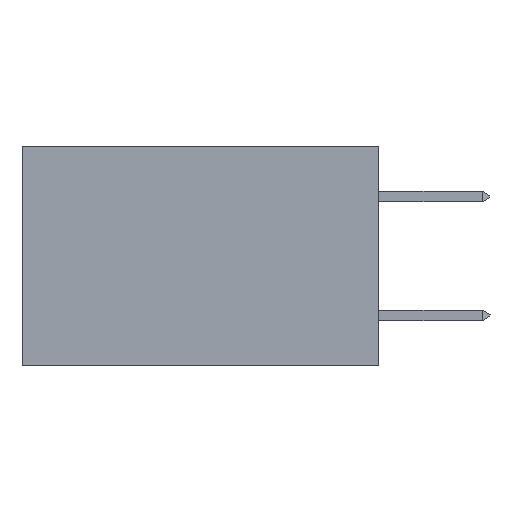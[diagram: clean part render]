
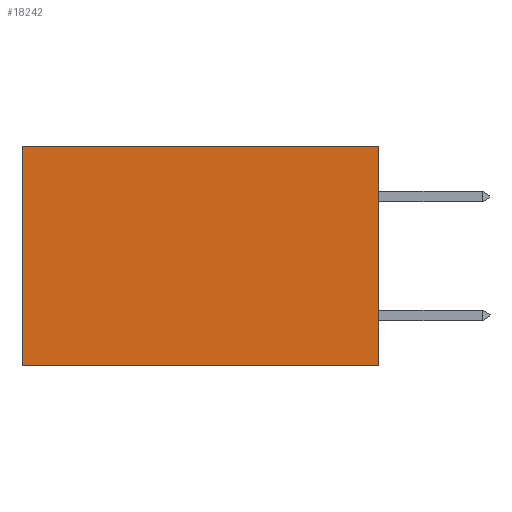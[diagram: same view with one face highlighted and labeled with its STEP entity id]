
A CAD part, left-side view. The second image highlights one B-rep face of the part: STEP entity #18242.
In plain terms, the highlighted planar face has unit normal (-1, 0, 0).
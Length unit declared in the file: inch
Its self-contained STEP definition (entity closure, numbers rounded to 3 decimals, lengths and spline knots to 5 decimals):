
#259 = VERTEX_POINT ( 'NONE', #22582 ) ;
#713 = CARTESIAN_POINT ( 'NONE',  ( 0.298, 0., 0. ) ) ;
#2427 = DIRECTION ( 'NONE',  ( 0., 1., 0. ) ) ;
#2491 = ORIENTED_EDGE ( 'NONE', *, *, #16410, .F. ) ;
#2570 = LINE ( 'NONE', #713, #17708 ) ;
#2868 = EDGE_CURVE ( 'NONE', #259, #24643, #7795, .T. ) ;
#3709 = VECTOR ( 'NONE', #2427, 39.37008 ) ;
#3842 = CARTESIAN_POINT ( 'NONE',  ( 0.298, 0., 0. ) ) ;
#5286 = FACE_OUTER_BOUND ( 'NONE', #17323, .T. ) ;
#5884 = VERTEX_POINT ( 'NONE', #3842 ) ;
#6358 = CARTESIAN_POINT ( 'NONE',  ( 0.298, 0., -0.37 ) ) ;
#7116 = AXIS2_PLACEMENT_3D ( 'NONE', #25518, #19274, #10791 ) ;
#7795 = LINE ( 'NONE', #15834, #25269 ) ;
#8068 = CARTESIAN_POINT ( 'NONE',  ( 0.298, 0., 0. ) ) ;
#10046 = VERTEX_POINT ( 'NONE', #6358 ) ;
#10791 = DIRECTION ( 'NONE',  ( 0., 0., -1. ) ) ;
#10875 = CARTESIAN_POINT ( 'NONE',  ( 0.298, 0., -0.37 ) ) ;
#12385 = ORIENTED_EDGE ( 'NONE', *, *, #26839, .F. ) ;
#12561 = EDGE_CURVE ( 'NONE', #5884, #259, #2570, .T. ) ;
#14695 = ORIENTED_EDGE ( 'NONE', *, *, #2868, .T. ) ;
#14833 = PLANE ( 'NONE',  #7116 ) ;
#15834 = CARTESIAN_POINT ( 'NONE',  ( 0.298, 0.6, 0. ) ) ;
#16410 = EDGE_CURVE ( 'NONE', #10046, #24643, #21798, .T. ) ;
#16470 = DIRECTION ( 'NONE',  ( 0., 0., -1. ) ) ;
#17323 = EDGE_LOOP ( 'NONE', ( #14695, #2491, #12385, #21413 ) ) ;
#17708 = VECTOR ( 'NONE', #19185, 39.37008 ) ;
#18242 = ADVANCED_FACE ( 'NONE', ( #5286 ), #14833, .F. ) ;
#18474 = VECTOR ( 'NONE', #16470, 39.37008 ) ;
#19185 = DIRECTION ( 'NONE',  ( 0., 1., 0. ) ) ;
#19274 = DIRECTION ( 'NONE',  ( 1., 0., 0. ) ) ;
#21413 = ORIENTED_EDGE ( 'NONE', *, *, #12561, .T. ) ;
#21798 = LINE ( 'NONE', #10875, #3709 ) ;
#22582 = CARTESIAN_POINT ( 'NONE',  ( 0.298, 0.6, 0. ) ) ;
#24123 = DIRECTION ( 'NONE',  ( 0., 0., -1. ) ) ;
#24502 = CARTESIAN_POINT ( 'NONE',  ( 0.298, 0.6, -0.37 ) ) ;
#24643 = VERTEX_POINT ( 'NONE', #24502 ) ;
#24726 = LINE ( 'NONE', #8068, #18474 ) ;
#25269 = VECTOR ( 'NONE', #24123, 39.37008 ) ;
#25518 = CARTESIAN_POINT ( 'NONE',  ( 0.298, 0., 0. ) ) ;
#26839 = EDGE_CURVE ( 'NONE', #5884, #10046, #24726, .T. ) ;
